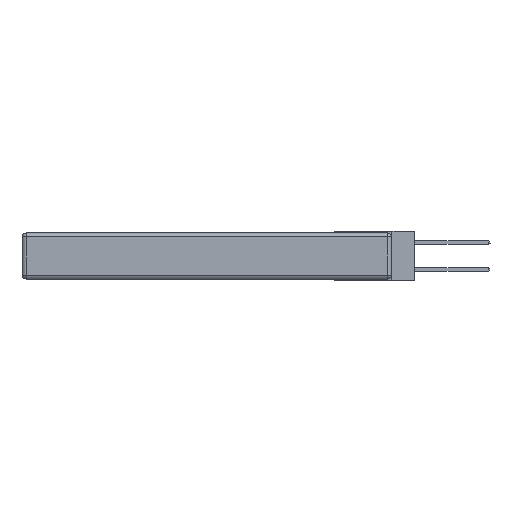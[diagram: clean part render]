
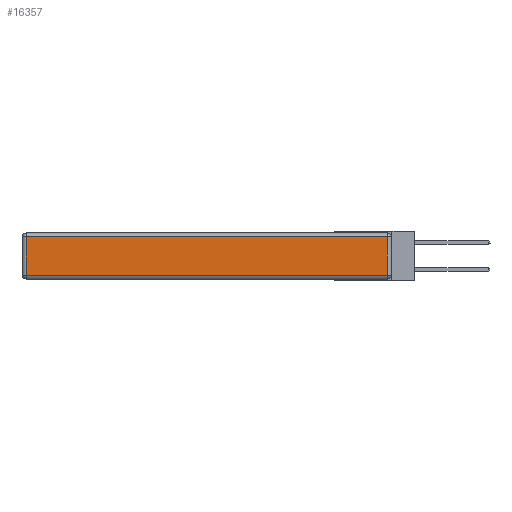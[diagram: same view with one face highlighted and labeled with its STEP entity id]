
A CAD part, left-side view. The second image highlights one B-rep face of the part: STEP entity #16357.
In plain terms, the highlighted planar face has unit normal (-1, 0, 0).
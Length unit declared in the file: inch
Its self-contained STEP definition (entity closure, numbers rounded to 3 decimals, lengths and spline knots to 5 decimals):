
#271 = VECTOR ( 'NONE', #469, 39.37008 ) ;
#469 = DIRECTION ( 'NONE',  ( 0., 1., 0. ) ) ;
#669 = VERTEX_POINT ( 'NONE', #19335 ) ;
#1739 = ORIENTED_EDGE ( 'NONE', *, *, #23563, .T. ) ;
#3169 = AXIS2_PLACEMENT_3D ( 'NONE', #16844, #6351, #8657 ) ;
#3677 = VERTEX_POINT ( 'NONE', #10056 ) ;
#6091 = ORIENTED_EDGE ( 'NONE', *, *, #23223, .T. ) ;
#6308 = CARTESIAN_POINT ( 'NONE',  ( 0., 2.72, -0.03 ) ) ;
#6351 = DIRECTION ( 'NONE',  ( -1., 0., 0. ) ) ;
#7003 = CARTESIAN_POINT ( 'NONE',  ( 0., 2.75, -0.03 ) ) ;
#7857 = LINE ( 'NONE', #7003, #271 ) ;
#7931 = EDGE_CURVE ( 'NONE', #3677, #13067, #13220, .T. ) ;
#8401 = VECTOR ( 'NONE', #19155, 39.37008 ) ;
#8657 = DIRECTION ( 'NONE',  ( 0., 0., 1. ) ) ;
#9457 = CARTESIAN_POINT ( 'NONE',  ( 0., 2.72, -0.343 ) ) ;
#9854 = EDGE_CURVE ( 'NONE', #26573, #669, #28123, .T. ) ;
#10049 = ORIENTED_EDGE ( 'NONE', *, *, #9854, .T. ) ;
#10056 = CARTESIAN_POINT ( 'NONE',  ( 0., 0.03, -0.313 ) ) ;
#10264 = FACE_OUTER_BOUND ( 'NONE', #16482, .T. ) ;
#13067 = VERTEX_POINT ( 'NONE', #18913 ) ;
#13220 = LINE ( 'NONE', #15557, #8401 ) ;
#13701 = LINE ( 'NONE', #21658, #14716 ) ;
#13890 = DIRECTION ( 'NONE',  ( 0., 0., -1. ) ) ;
#14716 = VECTOR ( 'NONE', #15131, 39.37008 ) ;
#15131 = DIRECTION ( 'NONE',  ( 0., -1., 0. ) ) ;
#15557 = CARTESIAN_POINT ( 'NONE',  ( 0., 0.03, -0.343 ) ) ;
#16117 = VECTOR ( 'NONE', #13890, 39.37008 ) ;
#16357 = ADVANCED_FACE ( 'NONE', ( #10264 ), #28192, .T. ) ;
#16482 = EDGE_LOOP ( 'NONE', ( #1739, #22849, #6091, #10049 ) ) ;
#16844 = CARTESIAN_POINT ( 'NONE',  ( 0., 0., -0.343 ) ) ;
#18913 = CARTESIAN_POINT ( 'NONE',  ( 0., 0.03, -0.03 ) ) ;
#19155 = DIRECTION ( 'NONE',  ( 0., 0., 1. ) ) ;
#19335 = CARTESIAN_POINT ( 'NONE',  ( 0., 2.72, -0.313 ) ) ;
#21658 = CARTESIAN_POINT ( 'NONE',  ( 0., 0., -0.313 ) ) ;
#22849 = ORIENTED_EDGE ( 'NONE', *, *, #7931, .T. ) ;
#23223 = EDGE_CURVE ( 'NONE', #13067, #26573, #7857, .T. ) ;
#23563 = EDGE_CURVE ( 'NONE', #669, #3677, #13701, .T. ) ;
#26573 = VERTEX_POINT ( 'NONE', #6308 ) ;
#28123 = LINE ( 'NONE', #9457, #16117 ) ;
#28192 = PLANE ( 'NONE',  #3169 ) ;
